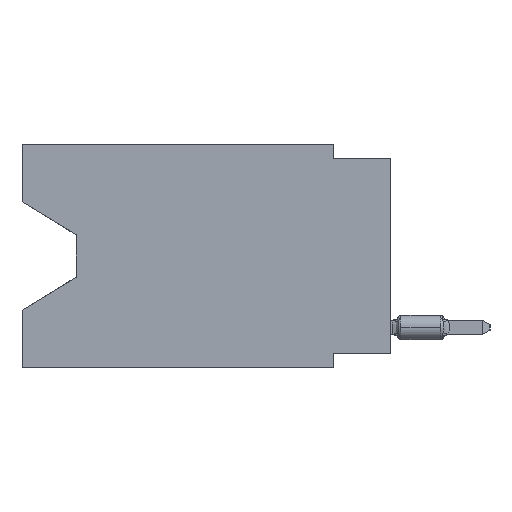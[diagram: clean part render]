
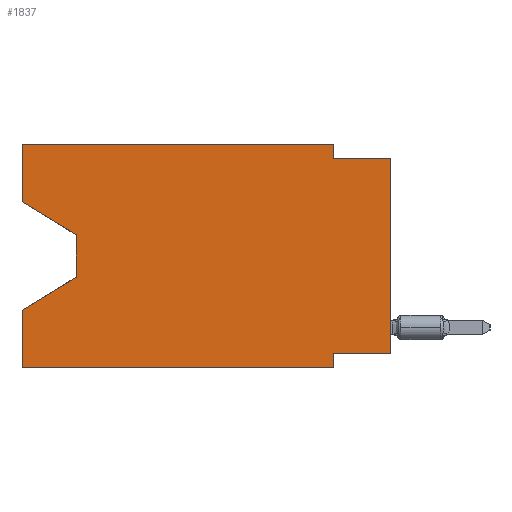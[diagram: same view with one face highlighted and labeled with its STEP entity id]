
A CAD part, left-side view. The second image highlights one B-rep face of the part: STEP entity #1837.
In plain terms, the highlighted planar face has unit normal (-1, 0, 0).
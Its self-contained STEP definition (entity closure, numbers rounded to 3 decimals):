
#239 = VERTEX_POINT ( 'NONE', #31664 ) ;
#668 = CARTESIAN_POINT ( 'NONE',  ( 0., 0., 0. ) ) ;
#1056 = ORIENTED_EDGE ( 'NONE', *, *, #34716, .F. ) ;
#1332 = VECTOR ( 'NONE', #1958, 1000. ) ;
#1837 = ADVANCED_FACE ( 'NONE', ( #8616 ), #21893, .F. ) ;
#1958 = DIRECTION ( 'NONE',  ( 0., 0., -1. ) ) ;
#2266 = EDGE_CURVE ( 'NONE', #20745, #6356, #33304, .T. ) ;
#2849 = CARTESIAN_POINT ( 'NONE',  ( 0., 16.383, 0. ) ) ;
#2916 = VERTEX_POINT ( 'NONE', #34258 ) ;
#4266 = CARTESIAN_POINT ( 'NONE',  ( 0., 2.54, -9.271 ) ) ;
#4291 = CARTESIAN_POINT ( 'NONE',  ( 0., 2.54, 0. ) ) ;
#4431 = ORIENTED_EDGE ( 'NONE', *, *, #28453, .F. ) ;
#4560 = DIRECTION ( 'NONE',  ( 0., 0., 1. ) ) ;
#5282 = ORIENTED_EDGE ( 'NONE', *, *, #9427, .T. ) ;
#5724 = ORIENTED_EDGE ( 'NONE', *, *, #20837, .F. ) ;
#5738 = VECTOR ( 'NONE', #29062, 1000. ) ;
#5786 = DIRECTION ( 'NONE',  ( 0., 0., -1. ) ) ;
#5839 = VECTOR ( 'NONE', #13751, 1000. ) ;
#6335 = ORIENTED_EDGE ( 'NONE', *, *, #13104, .F. ) ;
#6356 = VERTEX_POINT ( 'NONE', #22335 ) ;
#6509 = DIRECTION ( 'NONE',  ( 0., -1., 0. ) ) ;
#6746 = CARTESIAN_POINT ( 'NONE',  ( 0., 2.54, -0.635 ) ) ;
#7157 = AXIS2_PLACEMENT_3D ( 'NONE', #42278, #22328, #5786 ) ;
#7542 = DIRECTION ( 'NONE',  ( 0., 0., -1. ) ) ;
#7594 = LINE ( 'NONE', #13891, #11055 ) ;
#7770 = EDGE_CURVE ( 'NONE', #16276, #10366, #21952, .T. ) ;
#8616 = FACE_OUTER_BOUND ( 'NONE', #26960, .T. ) ;
#8921 = CARTESIAN_POINT ( 'NONE',  ( 0., 0., -0.635 ) ) ;
#9427 = EDGE_CURVE ( 'NONE', #41724, #6356, #30534, .T. ) ;
#9680 = VERTEX_POINT ( 'NONE', #6746 ) ;
#10114 = DIRECTION ( 'NONE',  ( 0., 1., 0. ) ) ;
#10310 = VECTOR ( 'NONE', #6509, 1000. ) ;
#10366 = VERTEX_POINT ( 'NONE', #34408 ) ;
#11055 = VECTOR ( 'NONE', #14101, 1000. ) ;
#11644 = LINE ( 'NONE', #12274, #30244 ) ;
#12274 = CARTESIAN_POINT ( 'NONE',  ( 0., 16.383, 0. ) ) ;
#12569 = VECTOR ( 'NONE', #10114, 1000. ) ;
#12603 = CARTESIAN_POINT ( 'NONE',  ( 0., 16.383, 0. ) ) ;
#13012 = DIRECTION ( 'NONE',  ( 0., -0.855, -0.519 ) ) ;
#13104 = EDGE_CURVE ( 'NONE', #31989, #9680, #24314, .T. ) ;
#13230 = LINE ( 'NONE', #33479, #26750 ) ;
#13419 = VECTOR ( 'NONE', #26763, 1000. ) ;
#13482 = CARTESIAN_POINT ( 'NONE',  ( 0., 2.54, -9.906 ) ) ;
#13751 = DIRECTION ( 'NONE',  ( 0., -1., 0. ) ) ;
#13891 = CARTESIAN_POINT ( 'NONE',  ( 0., 0., -0.635 ) ) ;
#14101 = DIRECTION ( 'NONE',  ( 0., -1., 0. ) ) ;
#15004 = VECTOR ( 'NONE', #35272, 1000. ) ;
#16276 = VERTEX_POINT ( 'NONE', #27780 ) ;
#16628 = CARTESIAN_POINT ( 'NONE',  ( 0., 2.54, 0. ) ) ;
#17014 = CARTESIAN_POINT ( 'NONE',  ( 0., 16.383, -9.906 ) ) ;
#18535 = ORIENTED_EDGE ( 'NONE', *, *, #24354, .T. ) ;
#20063 = CARTESIAN_POINT ( 'NONE',  ( 0., 16.383, 0. ) ) ;
#20745 = VERTEX_POINT ( 'NONE', #4266 ) ;
#20837 = EDGE_CURVE ( 'NONE', #239, #35388, #11644, .T. ) ;
#20861 = LINE ( 'NONE', #668, #36404 ) ;
#21389 = ORIENTED_EDGE ( 'NONE', *, *, #33230, .F. ) ;
#21674 = CARTESIAN_POINT ( 'NONE',  ( 0., 0., -9.271 ) ) ;
#21893 = PLANE ( 'NONE',  #7157 ) ;
#21952 = LINE ( 'NONE', #34360, #1332 ) ;
#22230 = CARTESIAN_POINT ( 'NONE',  ( 0., 13.97, -5.893 ) ) ;
#22328 = DIRECTION ( 'NONE',  ( 1., 0., 0. ) ) ;
#22335 = CARTESIAN_POINT ( 'NONE',  ( 0., 2.54, -9.906 ) ) ;
#23706 = EDGE_CURVE ( 'NONE', #10366, #2916, #25708, .T. ) ;
#24314 = LINE ( 'NONE', #4291, #28031 ) ;
#24354 = EDGE_CURVE ( 'NONE', #239, #16276, #13230, .T. ) ;
#25708 = LINE ( 'NONE', #22230, #15004 ) ;
#26750 = VECTOR ( 'NONE', #13012, 1000. ) ;
#26763 = DIRECTION ( 'NONE',  ( 0., 0., -1. ) ) ;
#26960 = EDGE_LOOP ( 'NONE', ( #18535, #32042, #29250, #1056, #5282, #38158, #21389, #34066, #28475, #6335, #4431, #5724 ) ) ;
#27780 = CARTESIAN_POINT ( 'NONE',  ( 0., 13.97, -4.013 ) ) ;
#28031 = VECTOR ( 'NONE', #7542, 1000. ) ;
#28453 = EDGE_CURVE ( 'NONE', #35388, #31989, #32638, .T. ) ;
#28475 = ORIENTED_EDGE ( 'NONE', *, *, #31319, .F. ) ;
#29045 = DIRECTION ( 'NONE',  ( 0., 0., 1. ) ) ;
#29062 = DIRECTION ( 'NONE',  ( 0., 0., 1. ) ) ;
#29214 = CARTESIAN_POINT ( 'NONE',  ( 0., 16.383, -9.906 ) ) ;
#29250 = ORIENTED_EDGE ( 'NONE', *, *, #23706, .T. ) ;
#30244 = VECTOR ( 'NONE', #29045, 1000. ) ;
#30534 = LINE ( 'NONE', #17014, #5839 ) ;
#31319 = EDGE_CURVE ( 'NONE', #9680, #35178, #7594, .T. ) ;
#31664 = CARTESIAN_POINT ( 'NONE',  ( 0., 16.383, -2.546 ) ) ;
#31989 = VERTEX_POINT ( 'NONE', #16628 ) ;
#32042 = ORIENTED_EDGE ( 'NONE', *, *, #7770, .T. ) ;
#32324 = LINE ( 'NONE', #20063, #5738 ) ;
#32638 = LINE ( 'NONE', #2849, #10310 ) ;
#33230 = EDGE_CURVE ( 'NONE', #38454, #20745, #39886, .T. ) ;
#33304 = LINE ( 'NONE', #13482, #13419 ) ;
#33479 = CARTESIAN_POINT ( 'NONE',  ( 0., 16.383, -2.546 ) ) ;
#34066 = ORIENTED_EDGE ( 'NONE', *, *, #36747, .T. ) ;
#34258 = CARTESIAN_POINT ( 'NONE',  ( 0., 16.383, -7.36 ) ) ;
#34360 = CARTESIAN_POINT ( 'NONE',  ( 0., 13.97, -4.013 ) ) ;
#34408 = CARTESIAN_POINT ( 'NONE',  ( 0., 13.97, -5.893 ) ) ;
#34716 = EDGE_CURVE ( 'NONE', #41724, #2916, #32324, .T. ) ;
#35178 = VERTEX_POINT ( 'NONE', #8921 ) ;
#35272 = DIRECTION ( 'NONE',  ( 0., 0.855, -0.519 ) ) ;
#35388 = VERTEX_POINT ( 'NONE', #12603 ) ;
#36404 = VECTOR ( 'NONE', #4560, 1000. ) ;
#36747 = EDGE_CURVE ( 'NONE', #38454, #35178, #20861, .T. ) ;
#38158 = ORIENTED_EDGE ( 'NONE', *, *, #2266, .F. ) ;
#38454 = VERTEX_POINT ( 'NONE', #21674 ) ;
#39886 = LINE ( 'NONE', #40103, #12569 ) ;
#40103 = CARTESIAN_POINT ( 'NONE',  ( 0., 0., -9.271 ) ) ;
#41724 = VERTEX_POINT ( 'NONE', #29214 ) ;
#42278 = CARTESIAN_POINT ( 'NONE',  ( 0., 16.383, 0. ) ) ;
